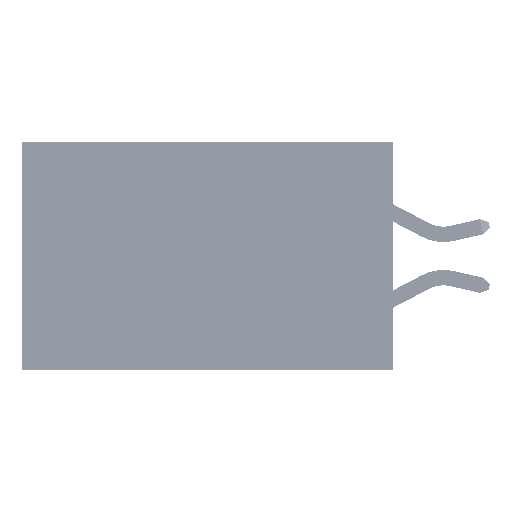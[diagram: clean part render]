
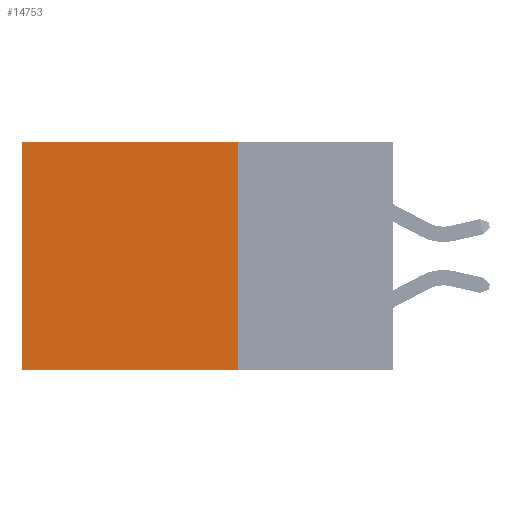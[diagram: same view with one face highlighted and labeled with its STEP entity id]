
A CAD part, left-side view. The second image highlights one B-rep face of the part: STEP entity #14753.
In plain terms, the highlighted planar face has unit normal (-1, 0, 0).
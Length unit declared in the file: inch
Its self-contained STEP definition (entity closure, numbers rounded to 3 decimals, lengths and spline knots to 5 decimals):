
#103 = FACE_OUTER_BOUND ( 'NONE', #26607, .T. ) ;
#620 = EDGE_CURVE ( 'NONE', #35831, #48031, #11130, .T. ) ;
#3314 = CARTESIAN_POINT ( 'NONE',  ( 0.2875, 0.25, 0. ) ) ;
#3619 = VECTOR ( 'NONE', #46218, 39.37008 ) ;
#3924 = LINE ( 'NONE', #27415, #31446 ) ;
#5460 = EDGE_CURVE ( 'NONE', #18995, #34710, #3924, .T. ) ;
#5587 = CARTESIAN_POINT ( 'NONE',  ( 0.2875, 0.25, 0. ) ) ;
#7594 = EDGE_CURVE ( 'NONE', #48031, #34710, #44255, .T. ) ;
#7930 = CARTESIAN_POINT ( 'NONE',  ( 0.2875, 0.25, 0. ) ) ;
#9667 = DIRECTION ( 'NONE',  ( 0., 0., -1. ) ) ;
#10035 = CARTESIAN_POINT ( 'NONE',  ( 0.2875, 0.25, -0.37 ) ) ;
#11130 = LINE ( 'NONE', #3314, #3619 ) ;
#13667 = ORIENTED_EDGE ( 'NONE', *, *, #5460, .F. ) ;
#14753 = ADVANCED_FACE ( 'NONE', ( #103 ), #34446, .F. ) ;
#15007 = DIRECTION ( 'NONE',  ( 0., 0., -1. ) ) ;
#18995 = VERTEX_POINT ( 'NONE', #10035 ) ;
#23365 = ORIENTED_EDGE ( 'NONE', *, *, #25613, .F. ) ;
#23719 = CARTESIAN_POINT ( 'NONE',  ( 0.2875, 0.25, 0. ) ) ;
#24570 = CARTESIAN_POINT ( 'NONE',  ( 0.2875, 0.6, 0. ) ) ;
#25595 = CARTESIAN_POINT ( 'NONE',  ( 0.2875, 0.6, 0. ) ) ;
#25613 = EDGE_CURVE ( 'NONE', #35831, #18995, #42898, .T. ) ;
#26607 = EDGE_LOOP ( 'NONE', ( #33713, #13667, #23365, #42619 ) ) ;
#26916 = DIRECTION ( 'NONE',  ( 0., 1., 0. ) ) ;
#27415 = CARTESIAN_POINT ( 'NONE',  ( 0.2875, 0.25, -0.37 ) ) ;
#28484 = VECTOR ( 'NONE', #39097, 39.37008 ) ;
#30164 = DIRECTION ( 'NONE',  ( 1., 0., 0. ) ) ;
#31446 = VECTOR ( 'NONE', #26916, 39.37008 ) ;
#32513 = AXIS2_PLACEMENT_3D ( 'NONE', #7930, #30164, #15007 ) ;
#33713 = ORIENTED_EDGE ( 'NONE', *, *, #7594, .T. ) ;
#34446 = PLANE ( 'NONE',  #32513 ) ;
#34710 = VERTEX_POINT ( 'NONE', #48051 ) ;
#35831 = VERTEX_POINT ( 'NONE', #5587 ) ;
#38551 = VECTOR ( 'NONE', #9667, 39.37008 ) ;
#39097 = DIRECTION ( 'NONE',  ( 0., 0., -1. ) ) ;
#42619 = ORIENTED_EDGE ( 'NONE', *, *, #620, .T. ) ;
#42898 = LINE ( 'NONE', #23719, #28484 ) ;
#44255 = LINE ( 'NONE', #25595, #38551 ) ;
#46218 = DIRECTION ( 'NONE',  ( 0., 1., 0. ) ) ;
#48031 = VERTEX_POINT ( 'NONE', #24570 ) ;
#48051 = CARTESIAN_POINT ( 'NONE',  ( 0.2875, 0.6, -0.37 ) ) ;
